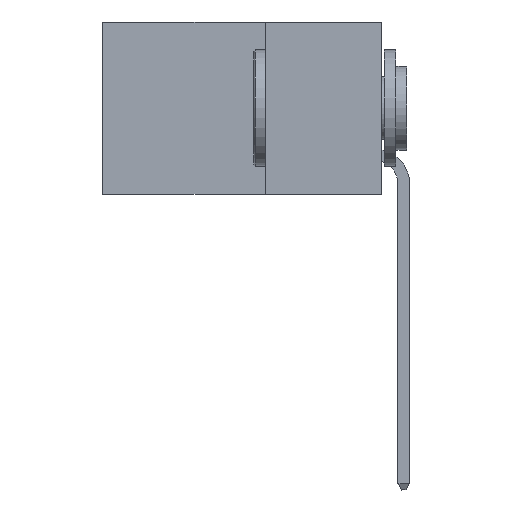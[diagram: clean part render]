
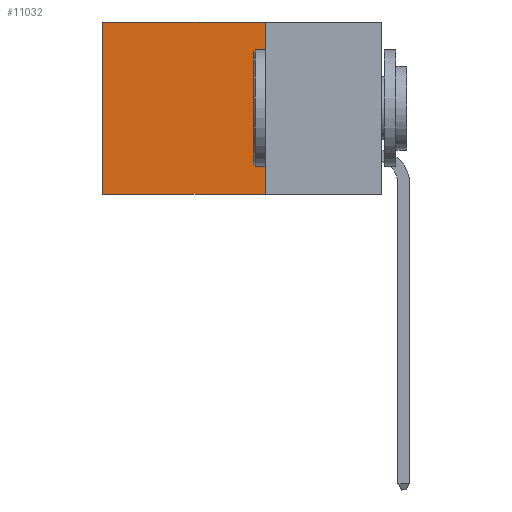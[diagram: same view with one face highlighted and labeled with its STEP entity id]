
A CAD part, left-side view. The second image highlights one B-rep face of the part: STEP entity #11032.
In plain terms, the highlighted planar face has unit normal (-1, 0, 0).
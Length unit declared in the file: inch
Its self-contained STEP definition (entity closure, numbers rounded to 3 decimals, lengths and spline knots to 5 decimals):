
#700 = VECTOR ( 'NONE', #23423, 39.37008 ) ;
#2409 = DIRECTION ( 'NONE',  ( 0., 1., 0. ) ) ;
#2683 = CARTESIAN_POINT ( 'NONE',  ( 0.2875, 0.6, -0.37 ) ) ;
#3590 = VECTOR ( 'NONE', #21257, 39.37008 ) ;
#6296 = CARTESIAN_POINT ( 'NONE',  ( 0.2875, 0.25, 0. ) ) ;
#7455 = AXIS2_PLACEMENT_3D ( 'NONE', #18841, #15427, #40665 ) ;
#7957 = CARTESIAN_POINT ( 'NONE',  ( 0.2875, 0.6, 0. ) ) ;
#11010 = VERTEX_POINT ( 'NONE', #22141 ) ;
#11032 = ADVANCED_FACE ( 'NONE', ( #36766 ), #31464, .F. ) ;
#11372 = CARTESIAN_POINT ( 'NONE',  ( 0.2875, 0.25, 0. ) ) ;
#14627 = LINE ( 'NONE', #7957, #700 ) ;
#15427 = DIRECTION ( 'NONE',  ( 1., 0., 0. ) ) ;
#16669 = EDGE_CURVE ( 'NONE', #34720, #24819, #20181, .T. ) ;
#17837 = VECTOR ( 'NONE', #2409, 39.37008 ) ;
#18215 = CARTESIAN_POINT ( 'NONE',  ( 0.2875, 0.25, 0. ) ) ;
#18382 = CARTESIAN_POINT ( 'NONE',  ( 0.2875, 0.25, -0.37 ) ) ;
#18841 = CARTESIAN_POINT ( 'NONE',  ( 0.2875, 0.25, 0. ) ) ;
#20181 = LINE ( 'NONE', #11372, #33106 ) ;
#21257 = DIRECTION ( 'NONE',  ( 0., 1., 0. ) ) ;
#21985 = EDGE_LOOP ( 'NONE', ( #28963, #26776, #36397, #22596 ) ) ;
#22141 = CARTESIAN_POINT ( 'NONE',  ( 0.2875, 0.6, 0. ) ) ;
#22596 = ORIENTED_EDGE ( 'NONE', *, *, #34468, .T. ) ;
#23423 = DIRECTION ( 'NONE',  ( 0., 0., -1. ) ) ;
#24819 = VERTEX_POINT ( 'NONE', #28546 ) ;
#26776 = ORIENTED_EDGE ( 'NONE', *, *, #38008, .F. ) ;
#27831 = LINE ( 'NONE', #18382, #3590 ) ;
#28546 = CARTESIAN_POINT ( 'NONE',  ( 0.2875, 0.25, -0.37 ) ) ;
#28963 = ORIENTED_EDGE ( 'NONE', *, *, #32119, .T. ) ;
#31464 = PLANE ( 'NONE',  #7455 ) ;
#32119 = EDGE_CURVE ( 'NONE', #11010, #38676, #14627, .T. ) ;
#33106 = VECTOR ( 'NONE', #40579, 39.37008 ) ;
#34468 = EDGE_CURVE ( 'NONE', #34720, #11010, #39578, .T. ) ;
#34720 = VERTEX_POINT ( 'NONE', #6296 ) ;
#36397 = ORIENTED_EDGE ( 'NONE', *, *, #16669, .F. ) ;
#36766 = FACE_OUTER_BOUND ( 'NONE', #21985, .T. ) ;
#38008 = EDGE_CURVE ( 'NONE', #24819, #38676, #27831, .T. ) ;
#38676 = VERTEX_POINT ( 'NONE', #2683 ) ;
#39578 = LINE ( 'NONE', #18215, #17837 ) ;
#40579 = DIRECTION ( 'NONE',  ( 0., 0., -1. ) ) ;
#40665 = DIRECTION ( 'NONE',  ( 0., 0., -1. ) ) ;
